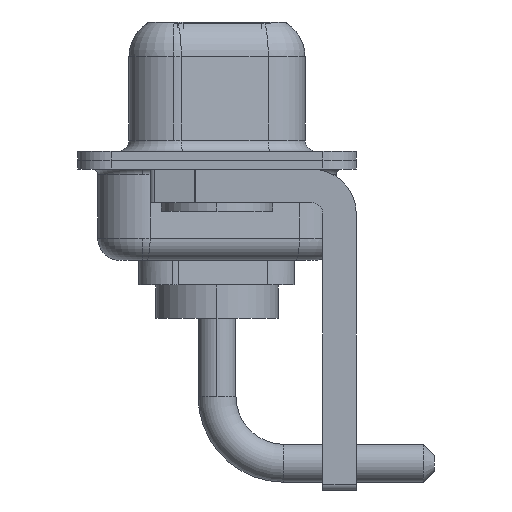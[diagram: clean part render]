
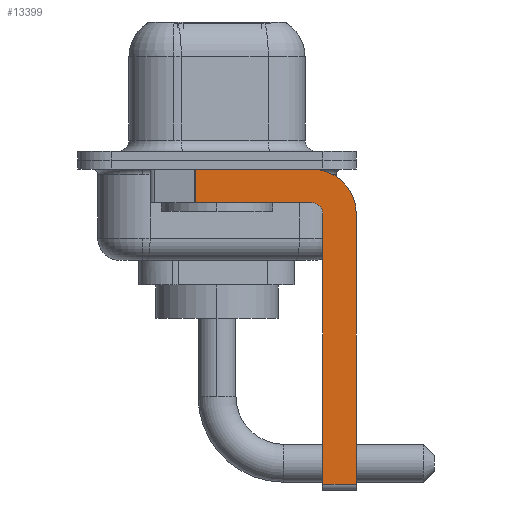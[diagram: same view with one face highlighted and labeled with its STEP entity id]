
A CAD part, left-side view. The second image highlights one B-rep face of the part: STEP entity #13399.
In plain terms, the highlighted planar face has unit normal (-1, 0, 0).
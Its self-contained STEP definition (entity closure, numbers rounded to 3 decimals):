
#96 = ORIENTED_EDGE ( 'NONE', *, *, #11246, .F. ) ;
#138 = LINE ( 'NONE', #10015, #9257 ) ;
#220 = DIRECTION ( 'NONE',  ( 0., -1., 0. ) ) ;
#557 = LINE ( 'NONE', #5098, #8858 ) ;
#966 = CARTESIAN_POINT ( 'NONE',  ( -2.9, -4.25, -1.9 ) ) ;
#1867 = ORIENTED_EDGE ( 'NONE', *, *, #3090, .F. ) ;
#1880 = CARTESIAN_POINT ( 'NONE',  ( -2.9, -4.25, -1.9 ) ) ;
#1946 = DIRECTION ( 'NONE',  ( 0., 0., -1. ) ) ;
#1993 = DIRECTION ( 'NONE',  ( 0., -1., 0. ) ) ;
#2115 = ORIENTED_EDGE ( 'NONE', *, *, #4627, .T. ) ;
#2509 = CARTESIAN_POINT ( 'NONE',  ( -2.9, -4.25, -0.4 ) ) ;
#2747 = EDGE_CURVE ( 'NONE', #9124, #8427, #10799, .T. ) ;
#2825 = CARTESIAN_POINT ( 'NONE',  ( -2.9, -6.25, -14.55 ) ) ;
#2996 = ORIENTED_EDGE ( 'NONE', *, *, #2747, .F. ) ;
#2997 = CARTESIAN_POINT ( 'NONE',  ( -2.9, -4.25, -2.4 ) ) ;
#3090 = EDGE_CURVE ( 'NONE', #8427, #10639, #4919, .T. ) ;
#3320 = CARTESIAN_POINT ( 'NONE',  ( -2.9, -4.75, -14.55 ) ) ;
#3514 = EDGE_CURVE ( 'NONE', #10125, #12771, #7178, .T. ) ;
#3544 = LINE ( 'NONE', #4615, #3796 ) ;
#3745 = DIRECTION ( 'NONE',  ( 0., 0., 1. ) ) ;
#3796 = VECTOR ( 'NONE', #4752, 1000. ) ;
#4074 = FACE_OUTER_BOUND ( 'NONE', #11132, .T. ) ;
#4615 = CARTESIAN_POINT ( 'NONE',  ( -2.9, -6.25, -2.4 ) ) ;
#4627 = EDGE_CURVE ( 'NONE', #5551, #10639, #13391, .T. ) ;
#4710 = VERTEX_POINT ( 'NONE', #2509 ) ;
#4752 = DIRECTION ( 'NONE',  ( 0., 0., -1. ) ) ;
#4919 = LINE ( 'NONE', #1880, #6051 ) ;
#5098 = CARTESIAN_POINT ( 'NONE',  ( -2.9, -4.75, -14.8 ) ) ;
#5551 = VERTEX_POINT ( 'NONE', #8003 ) ;
#5720 = CARTESIAN_POINT ( 'NONE',  ( -2.9, 0.978, -1.9 ) ) ;
#5800 = CARTESIAN_POINT ( 'NONE',  ( -2.9, -6.25, -2.4 ) ) ;
#6051 = VECTOR ( 'NONE', #9265, 1000. ) ;
#6275 = DIRECTION ( 'NONE',  ( 1., 0., 0. ) ) ;
#6722 = EDGE_CURVE ( 'NONE', #10125, #9124, #557, .T. ) ;
#7178 = LINE ( 'NONE', #11516, #11748 ) ;
#7798 = CARTESIAN_POINT ( 'NONE',  ( -2.9, 0.978, -1.9 ) ) ;
#8003 = CARTESIAN_POINT ( 'NONE',  ( -2.9, 0.978, -0.4 ) ) ;
#8071 = VERTEX_POINT ( 'NONE', #5800 ) ;
#8073 = DIRECTION ( 'NONE',  ( 0., 0., -1. ) ) ;
#8427 = VERTEX_POINT ( 'NONE', #966 ) ;
#8440 = CARTESIAN_POINT ( 'NONE',  ( -2.9, -4.25, -2.4 ) ) ;
#8858 = VECTOR ( 'NONE', #3745, 1000. ) ;
#9056 = ORIENTED_EDGE ( 'NONE', *, *, #3514, .T. ) ;
#9124 = VERTEX_POINT ( 'NONE', #9166 ) ;
#9166 = CARTESIAN_POINT ( 'NONE',  ( -2.9, -4.75, -2.4 ) ) ;
#9257 = VECTOR ( 'NONE', #220, 1000. ) ;
#9265 = DIRECTION ( 'NONE',  ( 0., 1., 0. ) ) ;
#9714 = AXIS2_PLACEMENT_3D ( 'NONE', #10343, #10212, #8073 ) ;
#10015 = CARTESIAN_POINT ( 'NONE',  ( -2.9, 3., -0.4 ) ) ;
#10125 = VERTEX_POINT ( 'NONE', #3320 ) ;
#10212 = DIRECTION ( 'NONE',  ( 1., 0., 0. ) ) ;
#10343 = CARTESIAN_POINT ( 'NONE',  ( -2.9, -4.25, -2.4 ) ) ;
#10639 = VERTEX_POINT ( 'NONE', #7798 ) ;
#10799 = CIRCLE ( 'NONE', #13751, 0.5 ) ;
#11079 = AXIS2_PLACEMENT_3D ( 'NONE', #2997, #6275, #1946 ) ;
#11132 = EDGE_LOOP ( 'NONE', ( #96, #2115, #1867, #2996, #13761, #9056, #13244, #12461 ) ) ;
#11246 = EDGE_CURVE ( 'NONE', #5551, #4710, #138, .T. ) ;
#11516 = CARTESIAN_POINT ( 'NONE',  ( -2.9, -4.25, -14.55 ) ) ;
#11640 = DIRECTION ( 'NONE',  ( 0., 0., 1. ) ) ;
#11748 = VECTOR ( 'NONE', #1993, 1000. ) ;
#11841 = EDGE_CURVE ( 'NONE', #4710, #8071, #12679, .T. ) ;
#12461 = ORIENTED_EDGE ( 'NONE', *, *, #11841, .F. ) ;
#12661 = EDGE_CURVE ( 'NONE', #8071, #12771, #3544, .T. ) ;
#12679 = CIRCLE ( 'NONE', #9714, 2. ) ;
#12749 = PLANE ( 'NONE',  #11079 ) ;
#12771 = VERTEX_POINT ( 'NONE', #2825 ) ;
#13115 = DIRECTION ( 'NONE',  ( 0., 0., -1. ) ) ;
#13244 = ORIENTED_EDGE ( 'NONE', *, *, #12661, .F. ) ;
#13391 = LINE ( 'NONE', #5720, #13576 ) ;
#13399 = ADVANCED_FACE ( 'NONE', ( #4074 ), #12749, .F. ) ;
#13576 = VECTOR ( 'NONE', #13115, 1000. ) ;
#13685 = DIRECTION ( 'NONE',  ( -1., 0., 0. ) ) ;
#13751 = AXIS2_PLACEMENT_3D ( 'NONE', #8440, #13685, #11640 ) ;
#13761 = ORIENTED_EDGE ( 'NONE', *, *, #6722, .F. ) ;
